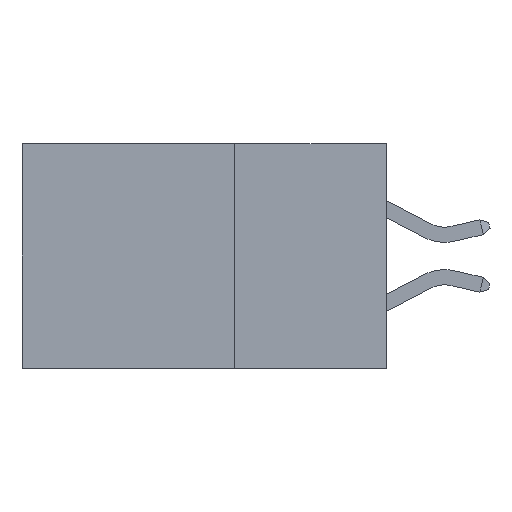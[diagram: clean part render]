
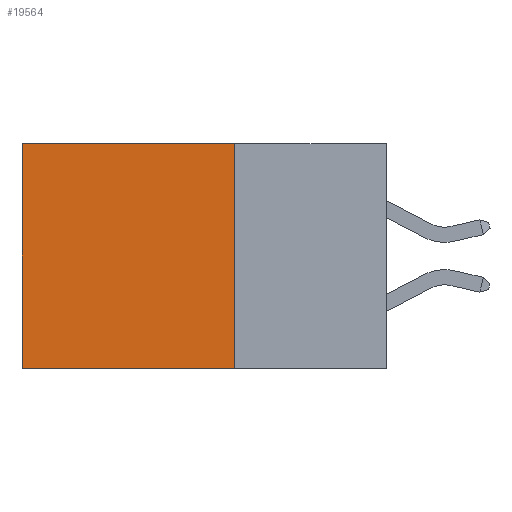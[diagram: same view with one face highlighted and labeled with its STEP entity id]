
A CAD part, left-side view. The second image highlights one B-rep face of the part: STEP entity #19564.
In plain terms, the highlighted planar face has unit normal (-1, 0, 0).
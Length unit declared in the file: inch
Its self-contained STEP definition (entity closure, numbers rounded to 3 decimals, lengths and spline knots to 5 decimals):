
#602 = CARTESIAN_POINT ( 'NONE',  ( 0.298, 0.25, -0.37 ) ) ;
#790 = LINE ( 'NONE', #4459, #20661 ) ;
#2006 = ORIENTED_EDGE ( 'NONE', *, *, #27077, .T. ) ;
#2252 = CARTESIAN_POINT ( 'NONE',  ( 0.298, 0.6, -0.37 ) ) ;
#4459 = CARTESIAN_POINT ( 'NONE',  ( 0.298, 0.6, 0. ) ) ;
#4558 = DIRECTION ( 'NONE',  ( 0., 0., -1. ) ) ;
#5041 = DIRECTION ( 'NONE',  ( 0., 0., -1. ) ) ;
#5803 = VERTEX_POINT ( 'NONE', #30974 ) ;
#6817 = VERTEX_POINT ( 'NONE', #9916 ) ;
#7284 = EDGE_LOOP ( 'NONE', ( #12470, #17397, #21315, #2006 ) ) ;
#7890 = EDGE_CURVE ( 'NONE', #5803, #29246, #22674, .T. ) ;
#8148 = VECTOR ( 'NONE', #16230, 39.37008 ) ;
#9619 = LINE ( 'NONE', #13183, #21674 ) ;
#9916 = CARTESIAN_POINT ( 'NONE',  ( 0.298, 0.25, 0. ) ) ;
#10234 = CARTESIAN_POINT ( 'NONE',  ( 0.298, 0.25, 0. ) ) ;
#10721 = EDGE_CURVE ( 'NONE', #28742, #29246, #790, .T. ) ;
#11084 = AXIS2_PLACEMENT_3D ( 'NONE', #10234, #20548, #5041 ) ;
#12470 = ORIENTED_EDGE ( 'NONE', *, *, #10721, .T. ) ;
#13183 = CARTESIAN_POINT ( 'NONE',  ( 0.298, 0.25, 0. ) ) ;
#13521 = EDGE_CURVE ( 'NONE', #6817, #5803, #9619, .T. ) ;
#16040 = CARTESIAN_POINT ( 'NONE',  ( 0.298, 0.6, 0. ) ) ;
#16230 = DIRECTION ( 'NONE',  ( 0., 1., 0. ) ) ;
#17397 = ORIENTED_EDGE ( 'NONE', *, *, #7890, .F. ) ;
#17471 = DIRECTION ( 'NONE',  ( 0., 1., 0. ) ) ;
#17485 = LINE ( 'NONE', #32807, #23500 ) ;
#17971 = PLANE ( 'NONE',  #11084 ) ;
#19564 = ADVANCED_FACE ( 'NONE', ( #24156 ), #17971, .F. ) ;
#20548 = DIRECTION ( 'NONE',  ( 1., 0., 0. ) ) ;
#20661 = VECTOR ( 'NONE', #4558, 39.37008 ) ;
#21315 = ORIENTED_EDGE ( 'NONE', *, *, #13521, .F. ) ;
#21674 = VECTOR ( 'NONE', #23521, 39.37008 ) ;
#22674 = LINE ( 'NONE', #602, #8148 ) ;
#23500 = VECTOR ( 'NONE', #17471, 39.37008 ) ;
#23521 = DIRECTION ( 'NONE',  ( 0., 0., -1. ) ) ;
#24156 = FACE_OUTER_BOUND ( 'NONE', #7284, .T. ) ;
#27077 = EDGE_CURVE ( 'NONE', #6817, #28742, #17485, .T. ) ;
#28742 = VERTEX_POINT ( 'NONE', #16040 ) ;
#29246 = VERTEX_POINT ( 'NONE', #2252 ) ;
#30974 = CARTESIAN_POINT ( 'NONE',  ( 0.298, 0.25, -0.37 ) ) ;
#32807 = CARTESIAN_POINT ( 'NONE',  ( 0.298, 0.25, 0. ) ) ;
